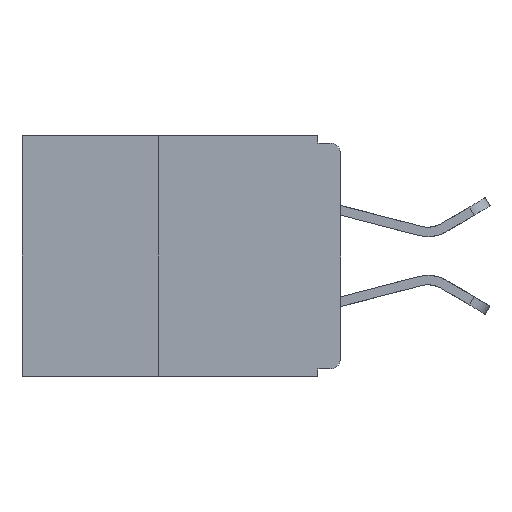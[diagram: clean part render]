
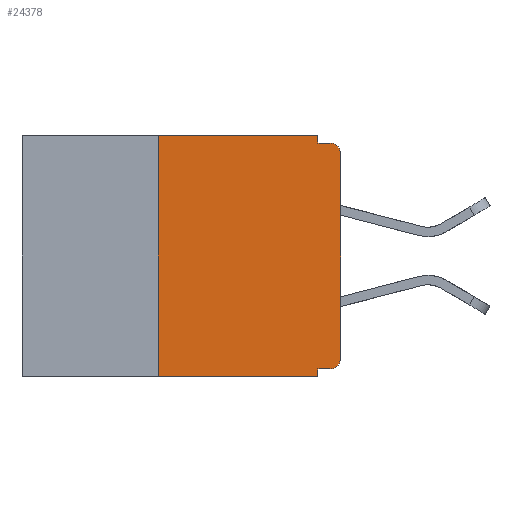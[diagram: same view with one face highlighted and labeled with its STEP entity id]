
A CAD part, left-side view. The second image highlights one B-rep face of the part: STEP entity #24378.
In plain terms, the highlighted planar face has unit normal (-1, 0, 0).
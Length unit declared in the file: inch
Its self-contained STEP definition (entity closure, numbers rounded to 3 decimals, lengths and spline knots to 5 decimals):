
#392 = ORIENTED_EDGE ( 'NONE', *, *, #17888, .F. ) ;
#864 = EDGE_CURVE ( 'NONE', #17817, #15750, #21967, .T. ) ;
#1470 = ORIENTED_EDGE ( 'NONE', *, *, #5516, .F. ) ;
#1711 = EDGE_CURVE ( 'NONE', #15750, #12412, #23640, .T. ) ;
#1952 = AXIS2_PLACEMENT_3D ( 'NONE', #15753, #4319, #17656 ) ;
#2023 = CARTESIAN_POINT ( 'NONE',  ( 0., 0., -0.32 ) ) ;
#2388 = ORIENTED_EDGE ( 'NONE', *, *, #11078, .T. ) ;
#2764 = CARTESIAN_POINT ( 'NONE',  ( 0., 0.031, -0.01 ) ) ;
#3613 = CIRCLE ( 'NONE', #1952, 0.015 ) ;
#3871 = ORIENTED_EDGE ( 'NONE', *, *, #9147, .F. ) ;
#4143 = CARTESIAN_POINT ( 'NONE',  ( 0., 0.031, -0.33 ) ) ;
#4235 = CARTESIAN_POINT ( 'NONE',  ( 0., 0., -0.01 ) ) ;
#4319 = DIRECTION ( 'NONE',  ( -1., 0., 0. ) ) ;
#4412 = DIRECTION ( 'NONE',  ( 0., -1., 0. ) ) ;
#4439 = VERTEX_POINT ( 'NONE', #20836 ) ;
#4525 = LINE ( 'NONE', #6323, #19121 ) ;
#4799 = VERTEX_POINT ( 'NONE', #14382 ) ;
#5395 = DIRECTION ( 'NONE',  ( 0., -1., 0. ) ) ;
#5516 = EDGE_CURVE ( 'NONE', #17607, #17817, #19560, .T. ) ;
#5756 = EDGE_LOOP ( 'NONE', ( #2388, #22431, #10335, #11574, #1470, #14917, #10397, #3871, #392, #15578 ) ) ;
#6323 = CARTESIAN_POINT ( 'NONE',  ( 0., 0.031, -0.33 ) ) ;
#6375 = CARTESIAN_POINT ( 'NONE',  ( 0., 0.437, -0.33 ) ) ;
#7094 = CARTESIAN_POINT ( 'NONE',  ( 0., 0.015, -0.305 ) ) ;
#7444 = VECTOR ( 'NONE', #8282, 39.37008 ) ;
#8223 = DIRECTION ( 'NONE',  ( 0., 0., -1. ) ) ;
#8282 = DIRECTION ( 'NONE',  ( 0., -1., 0. ) ) ;
#8756 = DIRECTION ( 'NONE',  ( 0., 0., -1. ) ) ;
#9021 = DIRECTION ( 'NONE',  ( 0., 0., -1. ) ) ;
#9147 = EDGE_CURVE ( 'NONE', #4799, #10921, #4525, .T. ) ;
#10189 = CARTESIAN_POINT ( 'NONE',  ( 0., 0., -0.305 ) ) ;
#10335 = ORIENTED_EDGE ( 'NONE', *, *, #1711, .F. ) ;
#10397 = ORIENTED_EDGE ( 'NONE', *, *, #21813, .T. ) ;
#10419 = CARTESIAN_POINT ( 'NONE',  ( 0., 0.031, 0. ) ) ;
#10443 = AXIS2_PLACEMENT_3D ( 'NONE', #12562, #20156, #8756 ) ;
#10921 = VERTEX_POINT ( 'NONE', #4143 ) ;
#11078 = EDGE_CURVE ( 'NONE', #19932, #17721, #12207, .T. ) ;
#11574 = ORIENTED_EDGE ( 'NONE', *, *, #864, .F. ) ;
#11790 = DIRECTION ( 'NONE',  ( 0., 0., -1. ) ) ;
#12207 = LINE ( 'NONE', #12318, #21680 ) ;
#12318 = CARTESIAN_POINT ( 'NONE',  ( 0., 0., 0. ) ) ;
#12388 = CARTESIAN_POINT ( 'NONE',  ( 0., 0.015, -0.32 ) ) ;
#12412 = VERTEX_POINT ( 'NONE', #14590 ) ;
#12562 = CARTESIAN_POINT ( 'NONE',  ( 0., 0.437, 0. ) ) ;
#14230 = DIRECTION ( 'NONE',  ( 0., 0., 1. ) ) ;
#14382 = CARTESIAN_POINT ( 'NONE',  ( 0., 0.031, -0.32 ) ) ;
#14535 = VECTOR ( 'NONE', #5395, 39.37008 ) ;
#14590 = CARTESIAN_POINT ( 'NONE',  ( 0., 0.015, -0.01 ) ) ;
#14917 = ORIENTED_EDGE ( 'NONE', *, *, #21045, .F. ) ;
#15272 = CIRCLE ( 'NONE', #24456, 0.015 ) ;
#15376 = DIRECTION ( 'NONE',  ( 0., 1., 0. ) ) ;
#15578 = ORIENTED_EDGE ( 'NONE', *, *, #21410, .T. ) ;
#15750 = VERTEX_POINT ( 'NONE', #2764 ) ;
#15753 = CARTESIAN_POINT ( 'NONE',  ( 0., 0.015, -0.025 ) ) ;
#15795 = VERTEX_POINT ( 'NONE', #12388 ) ;
#16466 = CARTESIAN_POINT ( 'NONE',  ( 0., 0.25, 0. ) ) ;
#16723 = CARTESIAN_POINT ( 'NONE',  ( 0., 0., -0.025 ) ) ;
#16770 = CARTESIAN_POINT ( 'NONE',  ( 0., 0.437, 0. ) ) ;
#17049 = LINE ( 'NONE', #6375, #7444 ) ;
#17503 = DIRECTION ( 'NONE',  ( 0., 0., 1. ) ) ;
#17512 = VECTOR ( 'NONE', #4412, 39.37008 ) ;
#17607 = VERTEX_POINT ( 'NONE', #16466 ) ;
#17656 = DIRECTION ( 'NONE',  ( 0., 0., -1. ) ) ;
#17721 = VERTEX_POINT ( 'NONE', #16723 ) ;
#17817 = VERTEX_POINT ( 'NONE', #18929 ) ;
#17888 = EDGE_CURVE ( 'NONE', #15795, #4799, #19695, .T. ) ;
#18855 = VECTOR ( 'NONE', #17503, 39.37008 ) ;
#18929 = CARTESIAN_POINT ( 'NONE',  ( 0., 0.031, 0. ) ) ;
#19103 = VECTOR ( 'NONE', #15376, 39.37008 ) ;
#19121 = VECTOR ( 'NONE', #8223, 39.37008 ) ;
#19435 = LINE ( 'NONE', #23057, #18855 ) ;
#19535 = FACE_OUTER_BOUND ( 'NONE', #5756, .T. ) ;
#19560 = LINE ( 'NONE', #16770, #14535 ) ;
#19695 = LINE ( 'NONE', #2023, #19103 ) ;
#19932 = VERTEX_POINT ( 'NONE', #10189 ) ;
#20078 = PLANE ( 'NONE',  #10443 ) ;
#20156 = DIRECTION ( 'NONE',  ( 1., 0., 0. ) ) ;
#20440 = DIRECTION ( 'NONE',  ( -1., 0., 0. ) ) ;
#20836 = CARTESIAN_POINT ( 'NONE',  ( 0., 0.25, -0.33 ) ) ;
#21045 = EDGE_CURVE ( 'NONE', #4439, #17607, #19435, .T. ) ;
#21377 = VECTOR ( 'NONE', #11790, 39.37008 ) ;
#21410 = EDGE_CURVE ( 'NONE', #15795, #19932, #15272, .T. ) ;
#21680 = VECTOR ( 'NONE', #14230, 39.37008 ) ;
#21740 = EDGE_CURVE ( 'NONE', #17721, #12412, #3613, .T. ) ;
#21813 = EDGE_CURVE ( 'NONE', #4439, #10921, #17049, .T. ) ;
#21967 = LINE ( 'NONE', #10419, #21377 ) ;
#22431 = ORIENTED_EDGE ( 'NONE', *, *, #21740, .T. ) ;
#23057 = CARTESIAN_POINT ( 'NONE',  ( 0., 0.25, -0.33 ) ) ;
#23640 = LINE ( 'NONE', #4235, #17512 ) ;
#24378 = ADVANCED_FACE ( 'NONE', ( #19535 ), #20078, .F. ) ;
#24456 = AXIS2_PLACEMENT_3D ( 'NONE', #7094, #20440, #9021 ) ;
